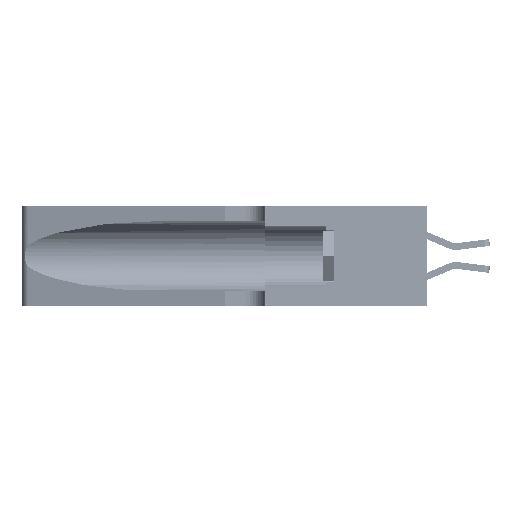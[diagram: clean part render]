
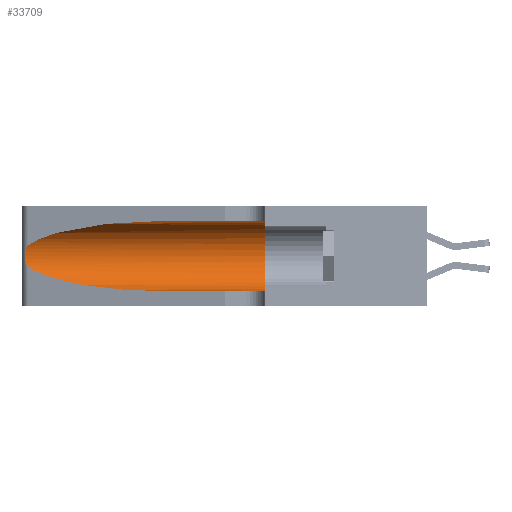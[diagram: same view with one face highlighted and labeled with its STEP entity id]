
A CAD part, left-side view. The second image highlights one B-rep face of the part: STEP entity #33709.
In plain terms, the highlighted cylindrical face has radius 3.308 mm (diameter 6.617 mm), a partial arc.
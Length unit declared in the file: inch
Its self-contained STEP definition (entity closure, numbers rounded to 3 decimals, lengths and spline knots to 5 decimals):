
#699 = EDGE_CURVE ( 'NONE', #8563, #43495, #4147, .T. ) ;
#849 = VERTEX_POINT ( 'NONE', #18846 ) ;
#945 = CARTESIAN_POINT ( 'NONE',  ( 0.1305, 1.61858, 0.185 ) ) ;
#1240 = CARTESIAN_POINT ( 'NONE',  ( 0.25487, 1.22718, 0.22369 ) ) ;
#3202 = CARTESIAN_POINT ( 'NONE',  ( 0.25639, 1.23186, 0.15144 ) ) ;
#3946 = EDGE_CURVE ( 'NONE', #39279, #849, #26342, .T. ) ;
#4147 = CIRCLE ( 'NONE', #15853, 0.13025 ) ;
#4506 = EDGE_CURVE ( 'NONE', #849, #11510, #9981, .T. ) ;
#6586 = CARTESIAN_POINT ( 'NONE',  ( 0.25487, 1.22718, 0.22369 ) ) ;
#6743 = CARTESIAN_POINT ( 'NONE',  ( 0.25487, 1.22718, 0.14631 ) ) ;
#7279 = CARTESIAN_POINT ( 'NONE',  ( 0.1305, 1.61858, 0.05475 ) ) ;
#7423 = ORIENTED_EDGE ( 'NONE', *, *, #13949, .F. ) ;
#8350 = CARTESIAN_POINT ( 'NONE',  ( 0.1305, 1.61858, 0.31525 ) ) ;
#8563 = VERTEX_POINT ( 'NONE', #45189 ) ;
#9654 = CARTESIAN_POINT ( 'NONE',  ( 0.25487, 1.22718, 0.14631 ) ) ;
#9661 = AXIS2_PLACEMENT_3D ( 'NONE', #945, #39344, #25631 ) ;
#9981 =( BOUNDED_CURVE ( )  B_SPLINE_CURVE ( 3, ( #9654, #30615, #37568, #16729 ),
 .UNSPECIFIED., .F., .T. ) 
 B_SPLINE_CURVE_WITH_KNOTS ( ( 4, 4 ),
 ( 3.44316, 4.71239 ),
 .UNSPECIFIED. ) 
 CURVE ( )  GEOMETRIC_REPRESENTATION_ITEM ( )  RATIONAL_B_SPLINE_CURVE ( ( 1., 0.87, 0.87, 1. ) ) 
 REPRESENTATION_ITEM ( '' )  );
#10166 = CARTESIAN_POINT ( 'NONE',  ( 0.25639, 1.23184, 0.21858 ) ) ;
#11510 = VERTEX_POINT ( 'NONE', #28387 ) ;
#11754 = CARTESIAN_POINT ( 'NONE',  ( 0.1305, 0.72297, 0.31525 ) ) ;
#12234 = ORIENTED_EDGE ( 'NONE', *, *, #699, .F. ) ;
#13717 = CARTESIAN_POINT ( 'NONE',  ( 0.25854, 1.2359, 0.20912 ) ) ;
#13949 = EDGE_CURVE ( 'NONE', #30533, #8563, #28624, .T. ) ;
#14030 = CYLINDRICAL_SURFACE ( 'NONE', #9661, 0.13025 ) ;
#15853 = AXIS2_PLACEMENT_3D ( 'NONE', #38901, #18081, #42356 ) ;
#16729 = CARTESIAN_POINT ( 'NONE',  ( 0.1305, 0.72297, 0.05475 ) ) ;
#17244 = CARTESIAN_POINT ( 'NONE',  ( 0.26075, 1.23896, 0.19203 ) ) ;
#18081 = DIRECTION ( 'NONE',  ( 0., 1., 0. ) ) ;
#18823 = CARTESIAN_POINT ( 'NONE',  ( 0.18966, 0.96281, 0.31525 ) ) ;
#18846 = CARTESIAN_POINT ( 'NONE',  ( 0.25487, 1.22718, 0.14631 ) ) ;
#18852 = CARTESIAN_POINT ( 'NONE',  ( 0.1305, 0.35, 0.05475 ) ) ;
#20797 = CARTESIAN_POINT ( 'NONE',  ( 0.26017, 1.23833, 0.17102 ) ) ;
#21870 = ORIENTED_EDGE ( 'NONE', *, *, #4506, .T. ) ;
#22408 = CARTESIAN_POINT ( 'NONE',  ( 0.2373, 1.15595, 0.28018 ) ) ;
#23699 = VECTOR ( 'NONE', #28329, 39.37008 ) ;
#24368 = CARTESIAN_POINT ( 'NONE',  ( 0.25789, 1.23486, 0.15765 ) ) ;
#25631 = DIRECTION ( 'NONE',  ( 0., 0., -1. ) ) ;
#26342 = B_SPLINE_CURVE_WITH_KNOTS ( 'NONE', 3,
 ( #6586, #27678, #10166, #34595, #13717, #38077, #17244, #41532, #20797, #44990, #24368, #3202, #27816, #6743 ),
 .UNSPECIFIED., .F., .F.,
 ( 4, 2, 2, 2, 2, 2, 4 ),
 ( 0., 0.00027, 0.00053, 0.00107, 0.0016, 0.00187, 0.00214 ),
 .UNSPECIFIED. ) ;
#26793 = EDGE_CURVE ( 'NONE', #11510, #43495, #42023, .T. ) ;
#26979 = EDGE_CURVE ( 'NONE', #30533, #39279, #35692, .T. ) ;
#27678 = CARTESIAN_POINT ( 'NONE',  ( 0.25555, 1.22994, 0.2215 ) ) ;
#27816 = CARTESIAN_POINT ( 'NONE',  ( 0.25555, 1.22993, 0.14849 ) ) ;
#28329 = DIRECTION ( 'NONE',  ( 0., -1., 0. ) ) ;
#28387 = CARTESIAN_POINT ( 'NONE',  ( 0.1305, 0.72297, 0.05475 ) ) ;
#28624 = LINE ( 'NONE', #8350, #36723 ) ;
#29160 = CARTESIAN_POINT ( 'NONE',  ( 0.25487, 1.22718, 0.22369 ) ) ;
#30533 = VERTEX_POINT ( 'NONE', #43218 ) ;
#30567 = ORIENTED_EDGE ( 'NONE', *, *, #26979, .T. ) ;
#30615 = CARTESIAN_POINT ( 'NONE',  ( 0.2373, 1.15595, 0.08982 ) ) ;
#32579 = FACE_OUTER_BOUND ( 'NONE', #37998, .T. ) ;
#33709 = ADVANCED_FACE ( 'NONE', ( #32579 ), #14030, .F. ) ;
#34595 = CARTESIAN_POINT ( 'NONE',  ( 0.25787, 1.23484, 0.2124 ) ) ;
#35692 =( BOUNDED_CURVE ( )  B_SPLINE_CURVE ( 3, ( #11754, #18823, #22408, #1240 ),
 .UNSPECIFIED., .F., .T. ) 
 B_SPLINE_CURVE_WITH_KNOTS ( ( 4, 4 ),
 ( 1.5708, 2.84003 ),
 .UNSPECIFIED. ) 
 CURVE ( )  GEOMETRIC_REPRESENTATION_ITEM ( )  RATIONAL_B_SPLINE_CURVE ( ( 1., 0.87, 0.87, 1. ) ) 
 REPRESENTATION_ITEM ( '' )  );
#36294 = DIRECTION ( 'NONE',  ( 0., -1., 0. ) ) ;
#36723 = VECTOR ( 'NONE', #36294, 39.37008 ) ;
#37112 = ORIENTED_EDGE ( 'NONE', *, *, #26793, .T. ) ;
#37568 = CARTESIAN_POINT ( 'NONE',  ( 0.18966, 0.96281, 0.05475 ) ) ;
#37998 = EDGE_LOOP ( 'NONE', ( #30567, #41949, #21870, #37112, #12234, #7423 ) ) ;
#38077 = CARTESIAN_POINT ( 'NONE',  ( 0.26018, 1.23835, 0.19895 ) ) ;
#38901 = CARTESIAN_POINT ( 'NONE',  ( 0.1305, 0.35, 0.185 ) ) ;
#39279 = VERTEX_POINT ( 'NONE', #29160 ) ;
#39344 = DIRECTION ( 'NONE',  ( 0., -1., 0. ) ) ;
#41532 = CARTESIAN_POINT ( 'NONE',  ( 0.26075, 1.23896, 0.178 ) ) ;
#41949 = ORIENTED_EDGE ( 'NONE', *, *, #3946, .T. ) ;
#42023 = LINE ( 'NONE', #7279, #23699 ) ;
#42356 = DIRECTION ( 'NONE',  ( 0., 0., 1. ) ) ;
#43218 = CARTESIAN_POINT ( 'NONE',  ( 0.1305, 0.72297, 0.31525 ) ) ;
#43495 = VERTEX_POINT ( 'NONE', #18852 ) ;
#44990 = CARTESIAN_POINT ( 'NONE',  ( 0.25856, 1.23593, 0.16098 ) ) ;
#45189 = CARTESIAN_POINT ( 'NONE',  ( 0.1305, 0.35, 0.31525 ) ) ;
